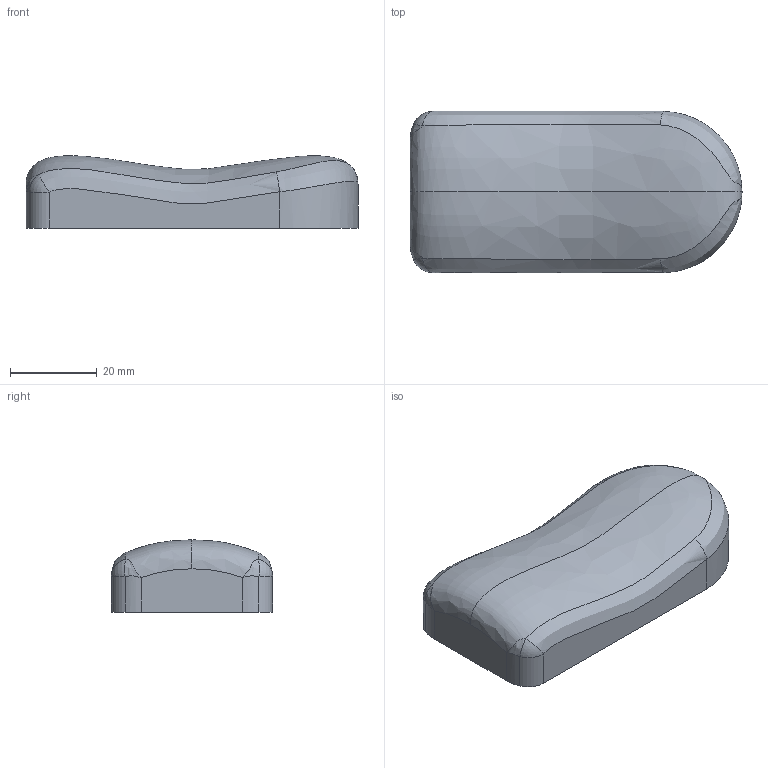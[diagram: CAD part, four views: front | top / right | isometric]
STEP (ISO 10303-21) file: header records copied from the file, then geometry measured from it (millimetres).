
FILE_DESCRIPTION (( 'STEP AP214' ), '1' );
FILE_NAME ('Butt_Pad.STEP', '2013-09-01T16:40:58', ( 'Asher' ), ( '' ), 'SwSTEP 2.0', 'SolidWorks 2013', '' );
FILE_SCHEMA (( 'AUTOMOTIVE_DESIGN' ));
Length unit declared in the file: millimetre
Products named in the file (1): Butt_Pad
Bounding box: 76.47 x 37.13 x 16.68 mm (x, y, z)
Volume: 36165.6 mm3; surface area: 8073.5 mm2
Topology: 1 solids, 1 shells, 25 faces, 60 edges, 33 vertices
Faces by surface type: cylinder 9, bspline 8, plane 6, sphere 2
Entity records: 1982 total; most frequent: CARTESIAN_POINT 1452, ORIENTED_EDGE 108, DIRECTION 93, EDGE_CURVE 54, AXIS2_PLACEMENT_3D 39, VERTEX_POINT 33, EDGE_LOOP 27, ADVANCED_FACE 25
